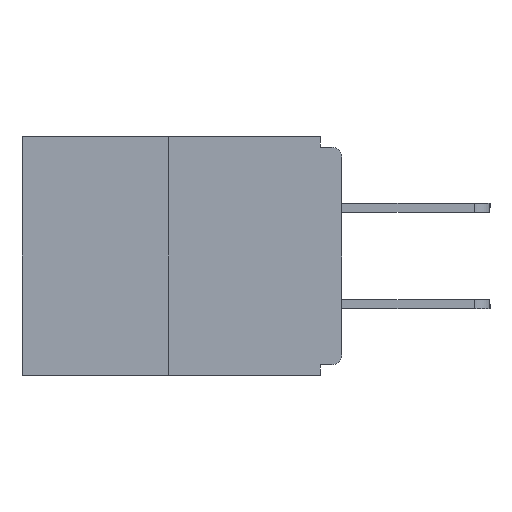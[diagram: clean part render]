
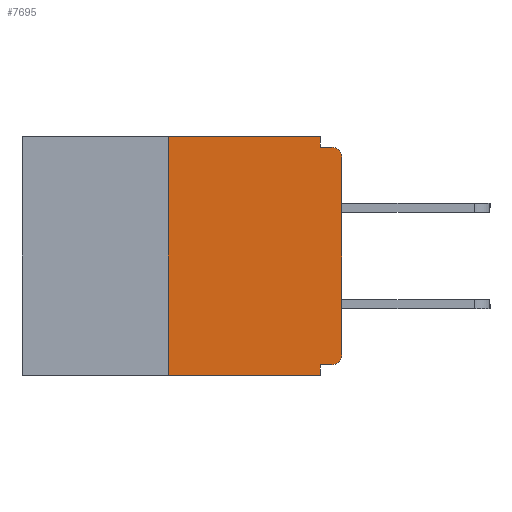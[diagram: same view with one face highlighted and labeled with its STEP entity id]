
A CAD part, left-side view. The second image highlights one B-rep face of the part: STEP entity #7695.
In plain terms, the highlighted planar face has unit normal (-1, 0, 0).
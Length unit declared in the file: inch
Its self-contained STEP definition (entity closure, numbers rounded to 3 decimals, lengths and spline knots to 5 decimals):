
#6 = DIRECTION ( 'NONE',  ( 0., 0., -1. ) ) ;
#187 = ORIENTED_EDGE ( 'NONE', *, *, #6152, .F. ) ;
#467 = VERTEX_POINT ( 'NONE', #8275 ) ;
#503 = ORIENTED_EDGE ( 'NONE', *, *, #8773, .T. ) ;
#959 = CARTESIAN_POINT ( 'NONE',  ( 0., 0.25, 0. ) ) ;
#1175 = CARTESIAN_POINT ( 'NONE',  ( 0., 0.015, -0.03 ) ) ;
#1185 = VERTEX_POINT ( 'NONE', #7603 ) ;
#1620 = ORIENTED_EDGE ( 'NONE', *, *, #12525, .F. ) ;
#1733 = CARTESIAN_POINT ( 'NONE',  ( 0., 0.031, -0.343 ) ) ;
#1788 = DIRECTION ( 'NONE',  ( 0., -1., 0. ) ) ;
#1870 = EDGE_CURVE ( 'NONE', #467, #8229, #12678, .T. ) ;
#1987 = CARTESIAN_POINT ( 'NONE',  ( 0., 0.031, -0.015 ) ) ;
#2001 = LINE ( 'NONE', #22286, #6284 ) ;
#2013 = DIRECTION ( 'NONE',  ( 0., 0., 1. ) ) ;
#2120 = VERTEX_POINT ( 'NONE', #10310 ) ;
#2795 = CIRCLE ( 'NONE', #20320, 0.015 ) ;
#3086 = VECTOR ( 'NONE', #10493, 39.37008 ) ;
#3230 = DIRECTION ( 'NONE',  ( 0., 0., 1. ) ) ;
#3446 = CARTESIAN_POINT ( 'NONE',  ( 0., 0.015, -0.328 ) ) ;
#3544 = CARTESIAN_POINT ( 'NONE',  ( 0., 0.25, 0. ) ) ;
#3717 = VECTOR ( 'NONE', #1788, 39.37008 ) ;
#3791 = CARTESIAN_POINT ( 'NONE',  ( 0., 0.46, -0.343 ) ) ;
#3945 = DIRECTION ( 'NONE',  ( 0., -1., 0. ) ) ;
#4020 = VECTOR ( 'NONE', #6, 39.37008 ) ;
#5201 = AXIS2_PLACEMENT_3D ( 'NONE', #14916, #20481, #6056 ) ;
#6056 = DIRECTION ( 'NONE',  ( 0., 0., -1. ) ) ;
#6152 = EDGE_CURVE ( 'NONE', #20355, #467, #21928, .T. ) ;
#6284 = VECTOR ( 'NONE', #3945, 39.37008 ) ;
#6329 = PLANE ( 'NONE',  #21185 ) ;
#6396 = EDGE_CURVE ( 'NONE', #21818, #22319, #6771, .T. ) ;
#6771 = LINE ( 'NONE', #12968, #10491 ) ;
#7056 = CARTESIAN_POINT ( 'NONE',  ( 0., 0., -0.015 ) ) ;
#7159 = LINE ( 'NONE', #3544, #21367 ) ;
#7592 = CARTESIAN_POINT ( 'NONE',  ( 0., 0.031, 0. ) ) ;
#7603 = CARTESIAN_POINT ( 'NONE',  ( 0., 0.015, -0.015 ) ) ;
#7695 = ADVANCED_FACE ( 'NONE', ( #16895 ), #6329, .F. ) ;
#7986 = ORIENTED_EDGE ( 'NONE', *, *, #19354, .F. ) ;
#8229 = VERTEX_POINT ( 'NONE', #19511 ) ;
#8275 = CARTESIAN_POINT ( 'NONE',  ( 0., 0.031, -0.328 ) ) ;
#8379 = DIRECTION ( 'NONE',  ( -1., 0., 0. ) ) ;
#8738 = EDGE_CURVE ( 'NONE', #9260, #11556, #7159, .T. ) ;
#8773 = EDGE_CURVE ( 'NONE', #9260, #8229, #10869, .T. ) ;
#9171 = CARTESIAN_POINT ( 'NONE',  ( 0., 0., -0.03 ) ) ;
#9260 = VERTEX_POINT ( 'NONE', #18286 ) ;
#9917 = EDGE_CURVE ( 'NONE', #20355, #21818, #15955, .T. ) ;
#10310 = CARTESIAN_POINT ( 'NONE',  ( 0., 0.031, 0. ) ) ;
#10491 = VECTOR ( 'NONE', #2013, 39.37008 ) ;
#10493 = DIRECTION ( 'NONE',  ( 0., 1., 0. ) ) ;
#10869 = LINE ( 'NONE', #3791, #3717 ) ;
#10901 = VECTOR ( 'NONE', #23517, 39.37008 ) ;
#11556 = VERTEX_POINT ( 'NONE', #959 ) ;
#11931 = DIRECTION ( 'NONE',  ( 1., 0., 0. ) ) ;
#12004 = DIRECTION ( 'NONE',  ( 0., 0., -1. ) ) ;
#12505 = ORIENTED_EDGE ( 'NONE', *, *, #23142, .T. ) ;
#12525 = EDGE_CURVE ( 'NONE', #22902, #1185, #21708, .T. ) ;
#12678 = LINE ( 'NONE', #1733, #17753 ) ;
#12968 = CARTESIAN_POINT ( 'NONE',  ( 0., 0., 0. ) ) ;
#13321 = ORIENTED_EDGE ( 'NONE', *, *, #18451, .F. ) ;
#14521 = DIRECTION ( 'NONE',  ( 0., 0., -1. ) ) ;
#14916 = CARTESIAN_POINT ( 'NONE',  ( 0., 0.015, -0.313 ) ) ;
#15955 = CIRCLE ( 'NONE', #5201, 0.015 ) ;
#16895 = FACE_OUTER_BOUND ( 'NONE', #23327, .T. ) ;
#17753 = VECTOR ( 'NONE', #14521, 39.37008 ) ;
#18286 = CARTESIAN_POINT ( 'NONE',  ( 0., 0.25, -0.343 ) ) ;
#18304 = ORIENTED_EDGE ( 'NONE', *, *, #6396, .T. ) ;
#18451 = EDGE_CURVE ( 'NONE', #11556, #2120, #2001, .T. ) ;
#19354 = EDGE_CURVE ( 'NONE', #2120, #22902, #23438, .T. ) ;
#19511 = CARTESIAN_POINT ( 'NONE',  ( 0., 0.031, -0.343 ) ) ;
#20320 = AXIS2_PLACEMENT_3D ( 'NONE', #1175, #8379, #21176 ) ;
#20355 = VERTEX_POINT ( 'NONE', #3446 ) ;
#20481 = DIRECTION ( 'NONE',  ( -1., 0., 0. ) ) ;
#21176 = DIRECTION ( 'NONE',  ( 0., 0., -1. ) ) ;
#21185 = AXIS2_PLACEMENT_3D ( 'NONE', #22866, #11931, #12004 ) ;
#21195 = ORIENTED_EDGE ( 'NONE', *, *, #1870, .F. ) ;
#21367 = VECTOR ( 'NONE', #3230, 39.37008 ) ;
#21708 = LINE ( 'NONE', #7056, #10901 ) ;
#21818 = VERTEX_POINT ( 'NONE', #22228 ) ;
#21906 = ORIENTED_EDGE ( 'NONE', *, *, #9917, .T. ) ;
#21928 = LINE ( 'NONE', #23034, #3086 ) ;
#22228 = CARTESIAN_POINT ( 'NONE',  ( 0., 0., -0.313 ) ) ;
#22286 = CARTESIAN_POINT ( 'NONE',  ( 0., 0.46, 0. ) ) ;
#22319 = VERTEX_POINT ( 'NONE', #9171 ) ;
#22866 = CARTESIAN_POINT ( 'NONE',  ( 0., 0.46, 0. ) ) ;
#22902 = VERTEX_POINT ( 'NONE', #1987 ) ;
#23034 = CARTESIAN_POINT ( 'NONE',  ( 0., 0., -0.328 ) ) ;
#23142 = EDGE_CURVE ( 'NONE', #22319, #1185, #2795, .T. ) ;
#23271 = ORIENTED_EDGE ( 'NONE', *, *, #8738, .F. ) ;
#23327 = EDGE_LOOP ( 'NONE', ( #13321, #23271, #503, #21195, #187, #21906, #18304, #12505, #1620, #7986 ) ) ;
#23438 = LINE ( 'NONE', #7592, #4020 ) ;
#23517 = DIRECTION ( 'NONE',  ( 0., -1., 0. ) ) ;
